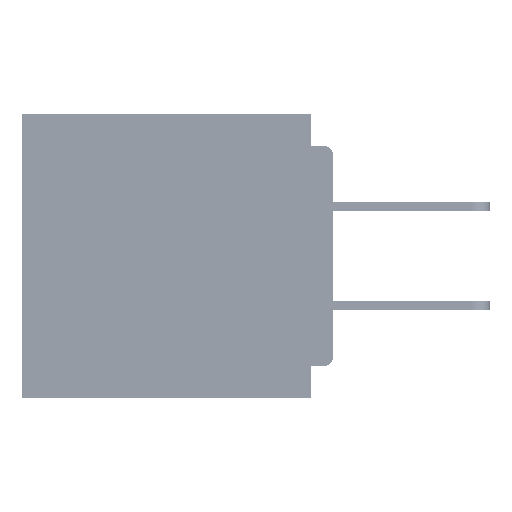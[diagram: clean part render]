
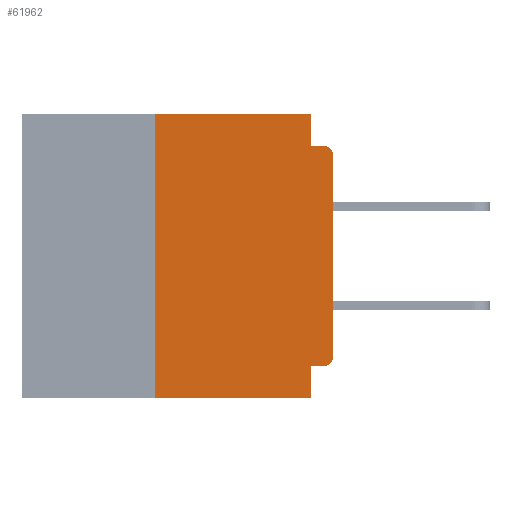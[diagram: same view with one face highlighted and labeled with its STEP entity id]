
A CAD part, left-side view. The second image highlights one B-rep face of the part: STEP entity #61962.
In plain terms, the highlighted planar face has unit normal (-1, 0, 0).
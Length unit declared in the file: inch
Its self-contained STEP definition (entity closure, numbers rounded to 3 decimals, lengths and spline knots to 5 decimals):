
#239 = CARTESIAN_POINT ( 'NONE',  ( 0., 0.031, 0. ) ) ;
#476 = CARTESIAN_POINT ( 'NONE',  ( 0., 0.25, 0. ) ) ;
#698 = ORIENTED_EDGE ( 'NONE', *, *, #26322, .F. ) ;
#1585 = DIRECTION ( 'NONE',  ( 0., -1., 0. ) ) ;
#2926 = CARTESIAN_POINT ( 'NONE',  ( 0., 0.25, -0.4 ) ) ;
#3561 = EDGE_CURVE ( 'NONE', #25034, #18071, #45656, .T. ) ;
#3613 = DIRECTION ( 'NONE',  ( 0., 0., -1. ) ) ;
#3915 = CARTESIAN_POINT ( 'NONE',  ( 0., 0.015, -0.06 ) ) ;
#4021 = EDGE_CURVE ( 'NONE', #55945, #28352, #6734, .T. ) ;
#4092 = VERTEX_POINT ( 'NONE', #23330 ) ;
#4221 = LINE ( 'NONE', #239, #54530 ) ;
#5669 = EDGE_CURVE ( 'NONE', #42165, #12596, #11092, .T. ) ;
#5876 = ORIENTED_EDGE ( 'NONE', *, *, #24203, .T. ) ;
#6734 = CIRCLE ( 'NONE', #30131, 0.015 ) ;
#6759 = DIRECTION ( 'NONE',  ( 0., 0., 1. ) ) ;
#7734 = EDGE_CURVE ( 'NONE', #42165, #23594, #35310, .T. ) ;
#8834 = DIRECTION ( 'NONE',  ( 0., 0., -1. ) ) ;
#9554 = VECTOR ( 'NONE', #42649, 39.37008 ) ;
#10476 = AXIS2_PLACEMENT_3D ( 'NONE', #42412, #32811, #3613 ) ;
#11092 = LINE ( 'NONE', #37750, #9554 ) ;
#11426 = FACE_OUTER_BOUND ( 'NONE', #55729, .T. ) ;
#12091 = ORIENTED_EDGE ( 'NONE', *, *, #3561, .T. ) ;
#12596 = VERTEX_POINT ( 'NONE', #476 ) ;
#13615 = CARTESIAN_POINT ( 'NONE',  ( 0., 0., -0.34 ) ) ;
#15562 = ORIENTED_EDGE ( 'NONE', *, *, #33229, .F. ) ;
#17212 = ORIENTED_EDGE ( 'NONE', *, *, #45444, .F. ) ;
#17242 = VERTEX_POINT ( 'NONE', #51188 ) ;
#18071 = VERTEX_POINT ( 'NONE', #13615 ) ;
#18299 = LINE ( 'NONE', #35724, #29742 ) ;
#20203 = CARTESIAN_POINT ( 'NONE',  ( 0., 0.015, -0.34 ) ) ;
#20263 = LINE ( 'NONE', #31073, #59068 ) ;
#23029 = PLANE ( 'NONE',  #10476 ) ;
#23330 = CARTESIAN_POINT ( 'NONE',  ( 0., 0.031, 0. ) ) ;
#23594 = VERTEX_POINT ( 'NONE', #60469 ) ;
#23859 = VECTOR ( 'NONE', #48786, 39.37008 ) ;
#24107 = CARTESIAN_POINT ( 'NONE',  ( 0., 0.015, -0.045 ) ) ;
#24203 = EDGE_CURVE ( 'NONE', #18071, #55945, #20263, .T. ) ;
#24795 = DIRECTION ( 'NONE',  ( 0., 0., -1. ) ) ;
#25034 = VERTEX_POINT ( 'NONE', #33198 ) ;
#25085 = DIRECTION ( 'NONE',  ( 0., 0., -1. ) ) ;
#25839 = DIRECTION ( 'NONE',  ( 0., 1., 0. ) ) ;
#26322 = EDGE_CURVE ( 'NONE', #34608, #28352, #62633, .T. ) ;
#27203 = EDGE_CURVE ( 'NONE', #12596, #4092, #18299, .T. ) ;
#27353 = CARTESIAN_POINT ( 'NONE',  ( 0., 0.031, -0.045 ) ) ;
#28352 = VERTEX_POINT ( 'NONE', #24107 ) ;
#28963 = ORIENTED_EDGE ( 'NONE', *, *, #7734, .T. ) ;
#29292 = ORIENTED_EDGE ( 'NONE', *, *, #27203, .F. ) ;
#29742 = VECTOR ( 'NONE', #1585, 39.37008 ) ;
#30131 = AXIS2_PLACEMENT_3D ( 'NONE', #3915, #38014, #8834 ) ;
#31073 = CARTESIAN_POINT ( 'NONE',  ( 0., 0., 0. ) ) ;
#31795 = LINE ( 'NONE', #45170, #56155 ) ;
#32811 = DIRECTION ( 'NONE',  ( 1., 0., 0. ) ) ;
#33198 = CARTESIAN_POINT ( 'NONE',  ( 0., 0.015, -0.355 ) ) ;
#33229 = EDGE_CURVE ( 'NONE', #17242, #23594, #38513, .T. ) ;
#34608 = VERTEX_POINT ( 'NONE', #27353 ) ;
#35310 = LINE ( 'NONE', #43229, #46710 ) ;
#35724 = CARTESIAN_POINT ( 'NONE',  ( 0., 0.437, 0. ) ) ;
#37750 = CARTESIAN_POINT ( 'NONE',  ( 0., 0.25, -0.4 ) ) ;
#37831 = ORIENTED_EDGE ( 'NONE', *, *, #5669, .F. ) ;
#38014 = DIRECTION ( 'NONE',  ( -1., 0., 0. ) ) ;
#38513 = LINE ( 'NONE', #52712, #49926 ) ;
#39029 = CARTESIAN_POINT ( 'NONE',  ( 0., 0., -0.045 ) ) ;
#41877 = ORIENTED_EDGE ( 'NONE', *, *, #4021, .T. ) ;
#42165 = VERTEX_POINT ( 'NONE', #2926 ) ;
#42412 = CARTESIAN_POINT ( 'NONE',  ( 0., 0.437, 0. ) ) ;
#42649 = DIRECTION ( 'NONE',  ( 0., 0., 1. ) ) ;
#42900 = ORIENTED_EDGE ( 'NONE', *, *, #57023, .F. ) ;
#43148 = DIRECTION ( 'NONE',  ( 0., 0., -1. ) ) ;
#43229 = CARTESIAN_POINT ( 'NONE',  ( 0., 0.437, -0.4 ) ) ;
#45170 = CARTESIAN_POINT ( 'NONE',  ( 0., 0., -0.355 ) ) ;
#45444 = EDGE_CURVE ( 'NONE', #4092, #34608, #4221, .T. ) ;
#45656 = CIRCLE ( 'NONE', #58640, 0.015 ) ;
#46710 = VECTOR ( 'NONE', #57877, 39.37008 ) ;
#48786 = DIRECTION ( 'NONE',  ( 0., -1., 0. ) ) ;
#49926 = VECTOR ( 'NONE', #43148, 39.37008 ) ;
#51188 = CARTESIAN_POINT ( 'NONE',  ( 0., 0.031, -0.355 ) ) ;
#52712 = CARTESIAN_POINT ( 'NONE',  ( 0., 0.031, -0.4 ) ) ;
#54229 = DIRECTION ( 'NONE',  ( -1., 0., 0. ) ) ;
#54530 = VECTOR ( 'NONE', #24795, 39.37008 ) ;
#55729 = EDGE_LOOP ( 'NONE', ( #5876, #41877, #698, #17212, #29292, #37831, #28963, #15562, #42900, #12091 ) ) ;
#55945 = VERTEX_POINT ( 'NONE', #59037 ) ;
#56155 = VECTOR ( 'NONE', #25839, 39.37008 ) ;
#57023 = EDGE_CURVE ( 'NONE', #25034, #17242, #31795, .T. ) ;
#57877 = DIRECTION ( 'NONE',  ( 0., -1., 0. ) ) ;
#58640 = AXIS2_PLACEMENT_3D ( 'NONE', #20203, #54229, #25085 ) ;
#59037 = CARTESIAN_POINT ( 'NONE',  ( 0., 0., -0.06 ) ) ;
#59068 = VECTOR ( 'NONE', #6759, 39.37008 ) ;
#60469 = CARTESIAN_POINT ( 'NONE',  ( 0., 0.031, -0.4 ) ) ;
#61962 = ADVANCED_FACE ( 'NONE', ( #11426 ), #23029, .F. ) ;
#62633 = LINE ( 'NONE', #39029, #23859 ) ;
